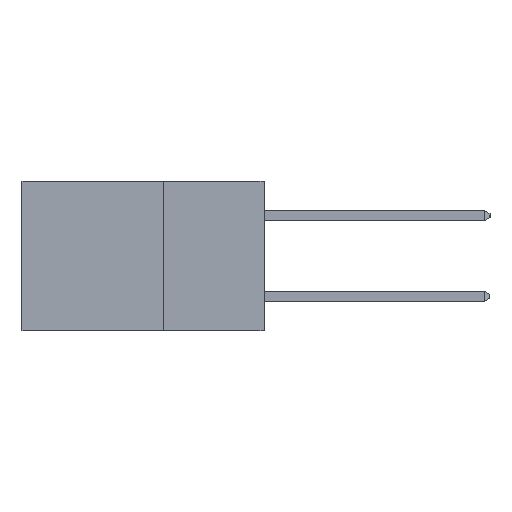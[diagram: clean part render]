
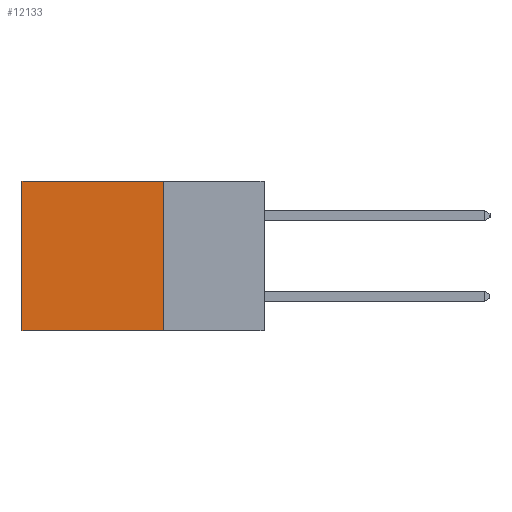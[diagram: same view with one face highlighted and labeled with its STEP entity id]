
A CAD part, left-side view. The second image highlights one B-rep face of the part: STEP entity #12133.
In plain terms, the highlighted planar face has unit normal (-1, 0, 0).
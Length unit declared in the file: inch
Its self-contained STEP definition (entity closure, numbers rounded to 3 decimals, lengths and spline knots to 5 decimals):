
#763 = VERTEX_POINT ( 'NONE', #797 ) ;
#776 = CARTESIAN_POINT ( 'NONE',  ( 0.298, 0.6, 0. ) ) ;
#797 = CARTESIAN_POINT ( 'NONE',  ( 0.298, 0.25, 0. ) ) ;
#1161 = LINE ( 'NONE', #7939, #11418 ) ;
#1472 = VECTOR ( 'NONE', #4479, 39.37008 ) ;
#1557 = DIRECTION ( 'NONE',  ( 1., 0., 0. ) ) ;
#1727 = CARTESIAN_POINT ( 'NONE',  ( 0.298, 0.25, 0. ) ) ;
#1799 = VERTEX_POINT ( 'NONE', #7053 ) ;
#2150 = DIRECTION ( 'NONE',  ( 0., 1., 0. ) ) ;
#2649 = VERTEX_POINT ( 'NONE', #11297 ) ;
#2700 = EDGE_CURVE ( 'NONE', #5437, #1799, #9019, .T. ) ;
#2919 = ORIENTED_EDGE ( 'NONE', *, *, #3815, .F. ) ;
#3257 = EDGE_CURVE ( 'NONE', #763, #5437, #5150, .T. ) ;
#3815 = EDGE_CURVE ( 'NONE', #2649, #1799, #4844, .T. ) ;
#3912 = ORIENTED_EDGE ( 'NONE', *, *, #3257, .T. ) ;
#4082 = AXIS2_PLACEMENT_3D ( 'NONE', #12084, #1557, #8177 ) ;
#4479 = DIRECTION ( 'NONE',  ( 0., 0., -1. ) ) ;
#4844 = LINE ( 'NONE', #6167, #6733 ) ;
#5120 = ORIENTED_EDGE ( 'NONE', *, *, #2700, .T. ) ;
#5150 = LINE ( 'NONE', #1727, #7586 ) ;
#5169 = ORIENTED_EDGE ( 'NONE', *, *, #6338, .F. ) ;
#5399 = EDGE_LOOP ( 'NONE', ( #5120, #2919, #5169, #3912 ) ) ;
#5437 = VERTEX_POINT ( 'NONE', #776 ) ;
#6167 = CARTESIAN_POINT ( 'NONE',  ( 0.298, 0.25, -0.37 ) ) ;
#6338 = EDGE_CURVE ( 'NONE', #763, #2649, #1161, .T. ) ;
#6733 = VECTOR ( 'NONE', #11181, 39.37008 ) ;
#7053 = CARTESIAN_POINT ( 'NONE',  ( 0.298, 0.6, -0.37 ) ) ;
#7275 = PLANE ( 'NONE',  #4082 ) ;
#7586 = VECTOR ( 'NONE', #2150, 39.37008 ) ;
#7939 = CARTESIAN_POINT ( 'NONE',  ( 0.298, 0.25, 0. ) ) ;
#8177 = DIRECTION ( 'NONE',  ( 0., 0., -1. ) ) ;
#9019 = LINE ( 'NONE', #9708, #1472 ) ;
#9108 = DIRECTION ( 'NONE',  ( 0., 0., -1. ) ) ;
#9705 = FACE_OUTER_BOUND ( 'NONE', #5399, .T. ) ;
#9708 = CARTESIAN_POINT ( 'NONE',  ( 0.298, 0.6, 0. ) ) ;
#11181 = DIRECTION ( 'NONE',  ( 0., 1., 0. ) ) ;
#11297 = CARTESIAN_POINT ( 'NONE',  ( 0.298, 0.25, -0.37 ) ) ;
#11418 = VECTOR ( 'NONE', #9108, 39.37008 ) ;
#12084 = CARTESIAN_POINT ( 'NONE',  ( 0.298, 0.25, 0. ) ) ;
#12133 = ADVANCED_FACE ( 'NONE', ( #9705 ), #7275, .F. ) ;
